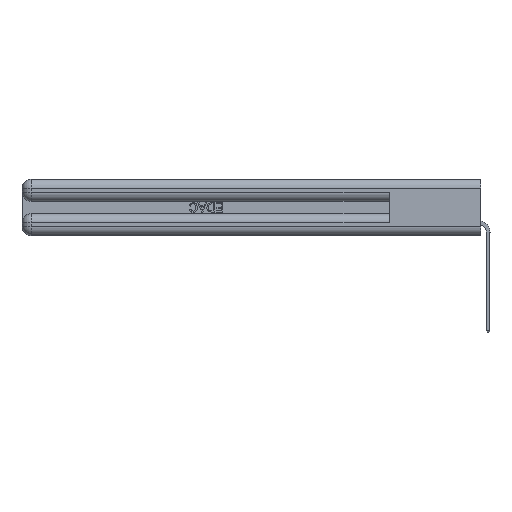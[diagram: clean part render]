
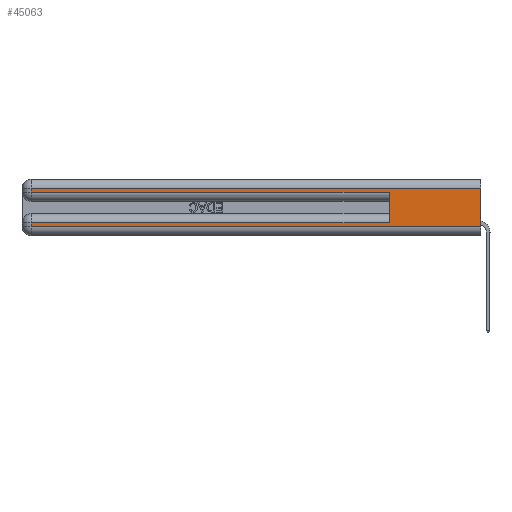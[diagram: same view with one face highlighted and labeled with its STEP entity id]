
A CAD part, left-side view. The second image highlights one B-rep face of the part: STEP entity #45063.
In plain terms, the highlighted planar face has unit normal (-1, 0, 0).
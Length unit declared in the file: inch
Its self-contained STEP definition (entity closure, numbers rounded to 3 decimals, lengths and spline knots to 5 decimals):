
#654 = ORIENTED_EDGE ( 'NONE', *, *, #38684, .F. ) ;
#1984 = VECTOR ( 'NONE', #9385, 39.37008 ) ;
#2862 = DIRECTION ( 'NONE',  ( 0., 0., 1. ) ) ;
#3130 = EDGE_LOOP ( 'NONE', ( #32889, #32993, #33678, #9821, #654, #34517, #20336, #16225 ) ) ;
#3827 = DIRECTION ( 'NONE',  ( 0., 0., -1. ) ) ;
#3873 = CARTESIAN_POINT ( 'NONE',  ( 0., 2.94, 0.085 ) ) ;
#5734 = DIRECTION ( 'NONE',  ( 0., 0., -1. ) ) ;
#7533 = VECTOR ( 'NONE', #26901, 39.37008 ) ;
#9385 = DIRECTION ( 'NONE',  ( 0., 0., -1. ) ) ;
#9821 = ORIENTED_EDGE ( 'NONE', *, *, #15963, .T. ) ;
#11125 = AXIS2_PLACEMENT_3D ( 'NONE', #28363, #40821, #3827 ) ;
#11276 = EDGE_CURVE ( 'NONE', #42546, #20310, #33253, .T. ) ;
#12729 = DIRECTION ( 'NONE',  ( 0., -1., 0. ) ) ;
#13955 = CARTESIAN_POINT ( 'NONE',  ( 0., 2.94, 0.06 ) ) ;
#14179 = EDGE_CURVE ( 'NONE', #21671, #20909, #20734, .T. ) ;
#15963 = EDGE_CURVE ( 'NONE', #51139, #24651, #35120, .T. ) ;
#16225 = ORIENTED_EDGE ( 'NONE', *, *, #45885, .T. ) ;
#17012 = VERTEX_POINT ( 'NONE', #17772 ) ;
#17772 = CARTESIAN_POINT ( 'NONE',  ( 0., 0.6, 0.085 ) ) ;
#18296 = LINE ( 'NONE', #51344, #7533 ) ;
#19957 = LINE ( 'NONE', #25735, #1984 ) ;
#20132 = CARTESIAN_POINT ( 'NONE',  ( 0., 2.94, 0.37 ) ) ;
#20310 = VERTEX_POINT ( 'NONE', #13955 ) ;
#20336 = ORIENTED_EDGE ( 'NONE', *, *, #11276, .T. ) ;
#20734 = LINE ( 'NONE', #30563, #49471 ) ;
#20909 = VERTEX_POINT ( 'NONE', #46274 ) ;
#21671 = VERTEX_POINT ( 'NONE', #37754 ) ;
#22349 = VECTOR ( 'NONE', #41380, 39.37008 ) ;
#22373 = LINE ( 'NONE', #30279, #51794 ) ;
#22845 = DIRECTION ( 'NONE',  ( 0., -1., 0. ) ) ;
#24378 = FACE_OUTER_BOUND ( 'NONE', #3130, .T. ) ;
#24651 = VERTEX_POINT ( 'NONE', #24726 ) ;
#24726 = CARTESIAN_POINT ( 'NONE',  ( 0., 0.6, 0.285 ) ) ;
#25735 = CARTESIAN_POINT ( 'NONE',  ( 0., 2.94, 0.37 ) ) ;
#26637 = DIRECTION ( 'NONE',  ( 0., 1., 0. ) ) ;
#26901 = DIRECTION ( 'NONE',  ( 0., 1., 0. ) ) ;
#28363 = CARTESIAN_POINT ( 'NONE',  ( 0., 0., 0.37 ) ) ;
#29055 = CARTESIAN_POINT ( 'NONE',  ( 0., 0., 0.285 ) ) ;
#29216 = VECTOR ( 'NONE', #2862, 39.37008 ) ;
#30279 = CARTESIAN_POINT ( 'NONE',  ( 0., 0., 0.37 ) ) ;
#30563 = CARTESIAN_POINT ( 'NONE',  ( 0., 0., 0.31 ) ) ;
#30667 = VECTOR ( 'NONE', #12729, 39.37008 ) ;
#32077 = EDGE_CURVE ( 'NONE', #17012, #42546, #18296, .T. ) ;
#32214 = CARTESIAN_POINT ( 'NONE',  ( 0., 0., 0.06 ) ) ;
#32889 = ORIENTED_EDGE ( 'NONE', *, *, #44658, .F. ) ;
#32993 = ORIENTED_EDGE ( 'NONE', *, *, #14179, .T. ) ;
#33253 = LINE ( 'NONE', #20132, #22349 ) ;
#33678 = ORIENTED_EDGE ( 'NONE', *, *, #48225, .T. ) ;
#34517 = ORIENTED_EDGE ( 'NONE', *, *, #32077, .T. ) ;
#35120 = LINE ( 'NONE', #29055, #30667 ) ;
#35645 = CARTESIAN_POINT ( 'NONE',  ( 0., 0.6, 0.145 ) ) ;
#36374 = VECTOR ( 'NONE', #22845, 39.37008 ) ;
#37538 = LINE ( 'NONE', #43195, #36374 ) ;
#37754 = CARTESIAN_POINT ( 'NONE',  ( 0., 0., 0.31 ) ) ;
#38684 = EDGE_CURVE ( 'NONE', #17012, #24651, #50919, .T. ) ;
#40821 = DIRECTION ( 'NONE',  ( 1., 0., 0. ) ) ;
#40986 = CARTESIAN_POINT ( 'NONE',  ( 0., 2.94, 0.285 ) ) ;
#41380 = DIRECTION ( 'NONE',  ( 0., 0., -1. ) ) ;
#42546 = VERTEX_POINT ( 'NONE', #3873 ) ;
#43195 = CARTESIAN_POINT ( 'NONE',  ( 0., 0., 0.06 ) ) ;
#44361 = VERTEX_POINT ( 'NONE', #32214 ) ;
#44658 = EDGE_CURVE ( 'NONE', #21671, #44361, #22373, .T. ) ;
#45063 = ADVANCED_FACE ( 'NONE', ( #24378 ), #45367, .F. ) ;
#45367 = PLANE ( 'NONE',  #11125 ) ;
#45885 = EDGE_CURVE ( 'NONE', #20310, #44361, #37538, .T. ) ;
#46274 = CARTESIAN_POINT ( 'NONE',  ( 0., 2.94, 0.31 ) ) ;
#48225 = EDGE_CURVE ( 'NONE', #20909, #51139, #19957, .T. ) ;
#49471 = VECTOR ( 'NONE', #26637, 39.37008 ) ;
#50919 = LINE ( 'NONE', #35645, #29216 ) ;
#51139 = VERTEX_POINT ( 'NONE', #40986 ) ;
#51344 = CARTESIAN_POINT ( 'NONE',  ( 0., 0., 0.085 ) ) ;
#51794 = VECTOR ( 'NONE', #5734, 39.37008 ) ;
